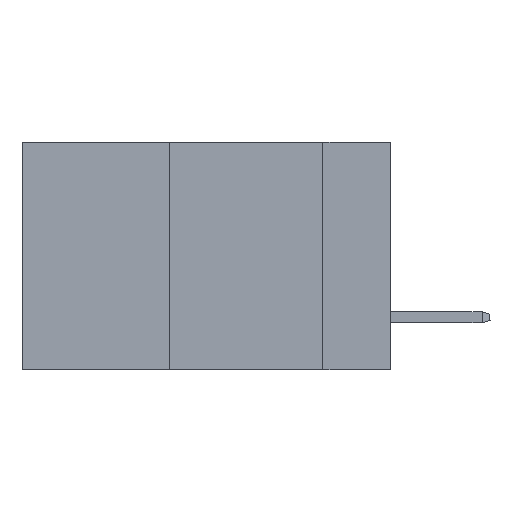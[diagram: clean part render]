
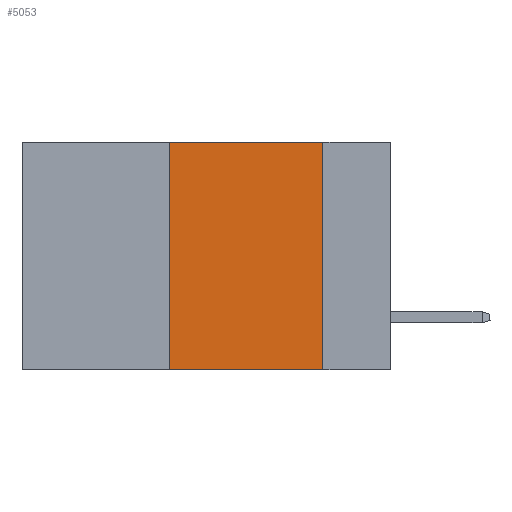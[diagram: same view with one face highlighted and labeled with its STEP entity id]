
A CAD part, left-side view. The second image highlights one B-rep face of the part: STEP entity #5053.
In plain terms, the highlighted planar face has unit normal (-1, 0, 0).
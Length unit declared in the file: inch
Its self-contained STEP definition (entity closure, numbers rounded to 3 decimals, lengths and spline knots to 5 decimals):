
#48 = VECTOR ( 'NONE', #6063, 39.37008 ) ;
#594 = LINE ( 'NONE', #8718, #10840 ) ;
#1428 = FACE_OUTER_BOUND ( 'NONE', #11394, .T. ) ;
#1558 = CARTESIAN_POINT ( 'NONE',  ( 0., 0.36, -0.37 ) ) ;
#1641 = LINE ( 'NONE', #7132, #48 ) ;
#1918 = VECTOR ( 'NONE', #7851, 39.37008 ) ;
#2131 = EDGE_CURVE ( 'NONE', #8675, #2752, #8114, .T. ) ;
#2196 = ORIENTED_EDGE ( 'NONE', *, *, #10382, .T. ) ;
#2412 = CARTESIAN_POINT ( 'NONE',  ( 0., 0.11, 0. ) ) ;
#2752 = VERTEX_POINT ( 'NONE', #4802 ) ;
#3053 = EDGE_CURVE ( 'NONE', #2752, #11774, #1641, .T. ) ;
#3080 = VECTOR ( 'NONE', #11345, 39.37008 ) ;
#3090 = DIRECTION ( 'NONE',  ( 0., 0., -1. ) ) ;
#4802 = CARTESIAN_POINT ( 'NONE',  ( 0., 0.36, 0. ) ) ;
#4858 = DIRECTION ( 'NONE',  ( 1., 0., 0. ) ) ;
#5053 = ADVANCED_FACE ( 'NONE', ( #1428 ), #8495, .F. ) ;
#5756 = CARTESIAN_POINT ( 'NONE',  ( 0., 0.6, 0. ) ) ;
#6063 = DIRECTION ( 'NONE',  ( 0., -1., 0. ) ) ;
#6511 = ORIENTED_EDGE ( 'NONE', *, *, #3053, .F. ) ;
#7132 = CARTESIAN_POINT ( 'NONE',  ( 0., 0.6, 0. ) ) ;
#7219 = CARTESIAN_POINT ( 'NONE',  ( 0., 0.11, -0.37 ) ) ;
#7246 = AXIS2_PLACEMENT_3D ( 'NONE', #5756, #4858, #10458 ) ;
#7851 = DIRECTION ( 'NONE',  ( 0., -1., 0. ) ) ;
#8114 = LINE ( 'NONE', #11209, #3080 ) ;
#8495 = PLANE ( 'NONE',  #7246 ) ;
#8675 = VERTEX_POINT ( 'NONE', #1558 ) ;
#8718 = CARTESIAN_POINT ( 'NONE',  ( 0., 0.11, 0. ) ) ;
#9520 = LINE ( 'NONE', #9917, #1918 ) ;
#9917 = CARTESIAN_POINT ( 'NONE',  ( 0., 0.6, -0.37 ) ) ;
#10023 = VERTEX_POINT ( 'NONE', #7219 ) ;
#10382 = EDGE_CURVE ( 'NONE', #8675, #10023, #9520, .T. ) ;
#10458 = DIRECTION ( 'NONE',  ( 0., 0., -1. ) ) ;
#10473 = ORIENTED_EDGE ( 'NONE', *, *, #2131, .F. ) ;
#10840 = VECTOR ( 'NONE', #3090, 39.37008 ) ;
#10844 = EDGE_CURVE ( 'NONE', #11774, #10023, #594, .T. ) ;
#10848 = ORIENTED_EDGE ( 'NONE', *, *, #10844, .F. ) ;
#11209 = CARTESIAN_POINT ( 'NONE',  ( 0., 0.36, 0. ) ) ;
#11345 = DIRECTION ( 'NONE',  ( 0., 0., 1. ) ) ;
#11394 = EDGE_LOOP ( 'NONE', ( #10848, #6511, #10473, #2196 ) ) ;
#11774 = VERTEX_POINT ( 'NONE', #2412 ) ;
